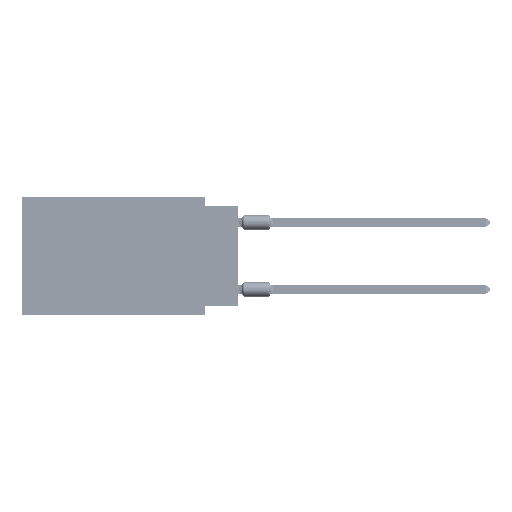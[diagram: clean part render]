
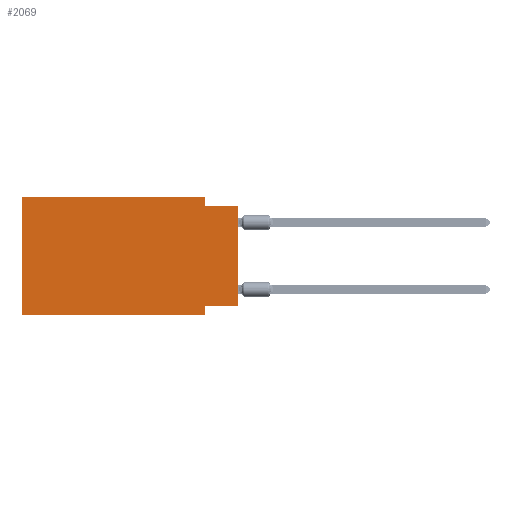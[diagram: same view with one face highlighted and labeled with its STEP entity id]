
A CAD part, left-side view. The second image highlights one B-rep face of the part: STEP entity #2069.
In plain terms, the highlighted planar face has unit normal (-1, 0, 0).
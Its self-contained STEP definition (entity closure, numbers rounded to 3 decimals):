
#1773 = ORIENTED_EDGE ( 'NONE', *, *, #10359, .F. ) ;
#2069 = ADVANCED_FACE ( 'NONE', ( #4290 ), #18945, .F. ) ;
#3480 = VECTOR ( 'NONE', #35062, 1000. ) ;
#4290 = FACE_OUTER_BOUND ( 'NONE', #70104, .T. ) ;
#4547 = CARTESIAN_POINT ( 'NONE',  ( 0., 0., -0.635 ) ) ;
#4923 = DIRECTION ( 'NONE',  ( 0., 0., -1. ) ) ;
#4988 = VERTEX_POINT ( 'NONE', #42439 ) ;
#5933 = CARTESIAN_POINT ( 'NONE',  ( 0., 2.54, -8.89 ) ) ;
#7566 = DIRECTION ( 'NONE',  ( 0., -1., 0. ) ) ;
#7588 = ORIENTED_EDGE ( 'NONE', *, *, #13474, .F. ) ;
#9780 = LINE ( 'NONE', #23990, #87099 ) ;
#10359 = EDGE_CURVE ( 'NONE', #71036, #4988, #33304, .T. ) ;
#10661 = DIRECTION ( 'NONE',  ( 0., 1., 0. ) ) ;
#11109 = EDGE_CURVE ( 'NONE', #71036, #15203, #36813, .T. ) ;
#12734 = EDGE_CURVE ( 'NONE', #56609, #76810, #18724, .T. ) ;
#13474 = EDGE_CURVE ( 'NONE', #55491, #88702, #9780, .T. ) ;
#15203 = VERTEX_POINT ( 'NONE', #60190 ) ;
#18142 = VERTEX_POINT ( 'NONE', #19019 ) ;
#18724 = LINE ( 'NONE', #67857, #79693 ) ;
#18945 = PLANE ( 'NONE',  #33336 ) ;
#19019 = CARTESIAN_POINT ( 'NONE',  ( 0., 0., -0.635 ) ) ;
#19606 = ORIENTED_EDGE ( 'NONE', *, *, #11109, .T. ) ;
#21357 = LINE ( 'NONE', #51183, #26605 ) ;
#21395 = EDGE_CURVE ( 'NONE', #55491, #18142, #29956, .T. ) ;
#23270 = EDGE_CURVE ( 'NONE', #88702, #15203, #61964, .T. ) ;
#23990 = CARTESIAN_POINT ( 'NONE',  ( 0., 0., -8.255 ) ) ;
#26605 = VECTOR ( 'NONE', #7566, 1000. ) ;
#28285 = ORIENTED_EDGE ( 'NONE', *, *, #12734, .F. ) ;
#29956 = LINE ( 'NONE', #69978, #3480 ) ;
#31840 = DIRECTION ( 'NONE',  ( 1., 0., 0. ) ) ;
#32551 = LINE ( 'NONE', #4547, #42185 ) ;
#32847 = DIRECTION ( 'NONE',  ( 0., 0., 1. ) ) ;
#33304 = LINE ( 'NONE', #47069, #52101 ) ;
#33336 = AXIS2_PLACEMENT_3D ( 'NONE', #46956, #31840, #38713 ) ;
#35062 = DIRECTION ( 'NONE',  ( 0., 0., 1. ) ) ;
#36813 = LINE ( 'NONE', #51071, #85537 ) ;
#37853 = ORIENTED_EDGE ( 'NONE', *, *, #21395, .T. ) ;
#38713 = DIRECTION ( 'NONE',  ( 0., 0., -1. ) ) ;
#41708 = ORIENTED_EDGE ( 'NONE', *, *, #55822, .F. ) ;
#42185 = VECTOR ( 'NONE', #65679, 1000. ) ;
#42439 = CARTESIAN_POINT ( 'NONE',  ( 0., 16.383, 0. ) ) ;
#42633 = CARTESIAN_POINT ( 'NONE',  ( 0., 16.383, -8.89 ) ) ;
#46021 = VECTOR ( 'NONE', #60612, 1000. ) ;
#46956 = CARTESIAN_POINT ( 'NONE',  ( 0., 16.383, 0. ) ) ;
#47069 = CARTESIAN_POINT ( 'NONE',  ( 0., 16.383, 0. ) ) ;
#51071 = CARTESIAN_POINT ( 'NONE',  ( 0., 16.383, -8.89 ) ) ;
#51183 = CARTESIAN_POINT ( 'NONE',  ( 0., 16.383, 0. ) ) ;
#52101 = VECTOR ( 'NONE', #32847, 1000. ) ;
#55491 = VERTEX_POINT ( 'NONE', #71522 ) ;
#55822 = EDGE_CURVE ( 'NONE', #4988, #56609, #21357, .T. ) ;
#56609 = VERTEX_POINT ( 'NONE', #64288 ) ;
#60190 = CARTESIAN_POINT ( 'NONE',  ( 0., 2.54, -8.89 ) ) ;
#60612 = DIRECTION ( 'NONE',  ( 0., 0., -1. ) ) ;
#61964 = LINE ( 'NONE', #5933, #46021 ) ;
#62858 = ORIENTED_EDGE ( 'NONE', *, *, #23270, .F. ) ;
#64288 = CARTESIAN_POINT ( 'NONE',  ( 0., 2.54, 0. ) ) ;
#64513 = ORIENTED_EDGE ( 'NONE', *, *, #77602, .F. ) ;
#65679 = DIRECTION ( 'NONE',  ( 0., -1., 0. ) ) ;
#66797 = CARTESIAN_POINT ( 'NONE',  ( 0., 2.54, -0.635 ) ) ;
#67857 = CARTESIAN_POINT ( 'NONE',  ( 0., 2.54, 0. ) ) ;
#69565 = CARTESIAN_POINT ( 'NONE',  ( 0., 2.54, -8.255 ) ) ;
#69978 = CARTESIAN_POINT ( 'NONE',  ( 0., 0., 0. ) ) ;
#70104 = EDGE_LOOP ( 'NONE', ( #37853, #64513, #28285, #41708, #1773, #19606, #62858, #7588 ) ) ;
#71036 = VERTEX_POINT ( 'NONE', #42633 ) ;
#71522 = CARTESIAN_POINT ( 'NONE',  ( 0., 0., -8.255 ) ) ;
#76810 = VERTEX_POINT ( 'NONE', #66797 ) ;
#77602 = EDGE_CURVE ( 'NONE', #76810, #18142, #32551, .T. ) ;
#78168 = DIRECTION ( 'NONE',  ( 0., -1., 0. ) ) ;
#79693 = VECTOR ( 'NONE', #4923, 1000. ) ;
#85537 = VECTOR ( 'NONE', #78168, 1000. ) ;
#87099 = VECTOR ( 'NONE', #10661, 1000. ) ;
#88702 = VERTEX_POINT ( 'NONE', #69565 ) ;
